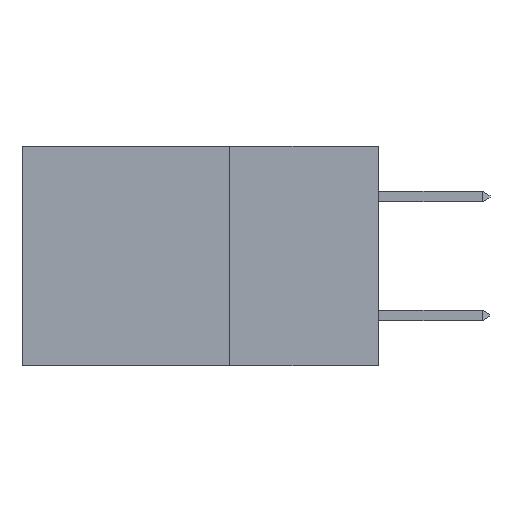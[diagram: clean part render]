
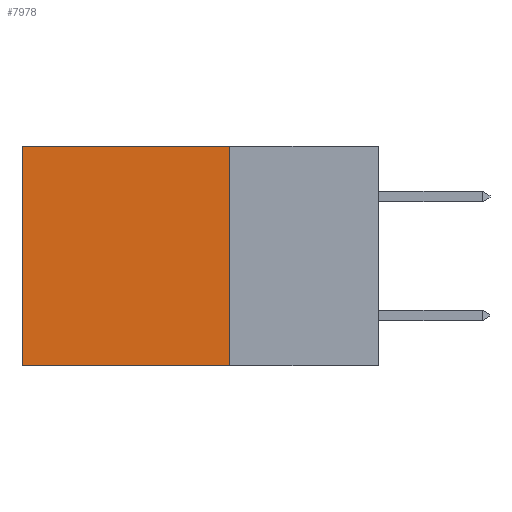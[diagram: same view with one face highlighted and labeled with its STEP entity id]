
A CAD part, left-side view. The second image highlights one B-rep face of the part: STEP entity #7978.
In plain terms, the highlighted planar face has unit normal (-1, 0, 0).
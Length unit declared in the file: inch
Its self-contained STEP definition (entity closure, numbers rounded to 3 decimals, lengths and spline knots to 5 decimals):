
#6 = CARTESIAN_POINT ( 'NONE',  ( 0.298, 0.6, 0. ) ) ;
#26 = VERTEX_POINT ( 'NONE', #4177 ) ;
#611 = FACE_OUTER_BOUND ( 'NONE', #9660, .T. ) ;
#937 = LINE ( 'NONE', #8434, #12042 ) ;
#1011 = LINE ( 'NONE', #7320, #4480 ) ;
#1591 = DIRECTION ( 'NONE',  ( 0., 1., 0. ) ) ;
#2080 = DIRECTION ( 'NONE',  ( 1., 0., 0. ) ) ;
#2185 = ORIENTED_EDGE ( 'NONE', *, *, #2963, .T. ) ;
#2963 = EDGE_CURVE ( 'NONE', #7010, #9437, #8367, .T. ) ;
#2979 = DIRECTION ( 'NONE',  ( 0., 0., -1. ) ) ;
#3249 = AXIS2_PLACEMENT_3D ( 'NONE', #13728, #2080, #9654 ) ;
#3336 = CARTESIAN_POINT ( 'NONE',  ( 0.298, 0.25, 0. ) ) ;
#3749 = EDGE_CURVE ( 'NONE', #9437, #26, #1011, .T. ) ;
#4085 = VECTOR ( 'NONE', #1591, 39.37008 ) ;
#4119 = DIRECTION ( 'NONE',  ( 0., 0., -1. ) ) ;
#4154 = ORIENTED_EDGE ( 'NONE', *, *, #9929, .F. ) ;
#4177 = CARTESIAN_POINT ( 'NONE',  ( 0.298, 0.6, -0.37 ) ) ;
#4480 = VECTOR ( 'NONE', #4119, 39.37008 ) ;
#5577 = ORIENTED_EDGE ( 'NONE', *, *, #5966, .F. ) ;
#5825 = CARTESIAN_POINT ( 'NONE',  ( 0.298, 0.25, -0.37 ) ) ;
#5841 = CARTESIAN_POINT ( 'NONE',  ( 0.298, 0.25, -0.37 ) ) ;
#5966 = EDGE_CURVE ( 'NONE', #12656, #26, #9946, .T. ) ;
#7010 = VERTEX_POINT ( 'NONE', #3336 ) ;
#7320 = CARTESIAN_POINT ( 'NONE',  ( 0.298, 0.6, 0. ) ) ;
#7978 = ADVANCED_FACE ( 'NONE', ( #611 ), #8572, .F. ) ;
#8367 = LINE ( 'NONE', #11324, #13853 ) ;
#8434 = CARTESIAN_POINT ( 'NONE',  ( 0.298, 0.25, 0. ) ) ;
#8526 = ORIENTED_EDGE ( 'NONE', *, *, #3749, .T. ) ;
#8572 = PLANE ( 'NONE',  #3249 ) ;
#9437 = VERTEX_POINT ( 'NONE', #6 ) ;
#9654 = DIRECTION ( 'NONE',  ( 0., 0., -1. ) ) ;
#9660 = EDGE_LOOP ( 'NONE', ( #8526, #5577, #4154, #2185 ) ) ;
#9929 = EDGE_CURVE ( 'NONE', #7010, #12656, #937, .T. ) ;
#9946 = LINE ( 'NONE', #5841, #4085 ) ;
#10959 = DIRECTION ( 'NONE',  ( 0., 1., 0. ) ) ;
#11324 = CARTESIAN_POINT ( 'NONE',  ( 0.298, 0.25, 0. ) ) ;
#12042 = VECTOR ( 'NONE', #2979, 39.37008 ) ;
#12656 = VERTEX_POINT ( 'NONE', #5825 ) ;
#13728 = CARTESIAN_POINT ( 'NONE',  ( 0.298, 0.25, 0. ) ) ;
#13853 = VECTOR ( 'NONE', #10959, 39.37008 ) ;
